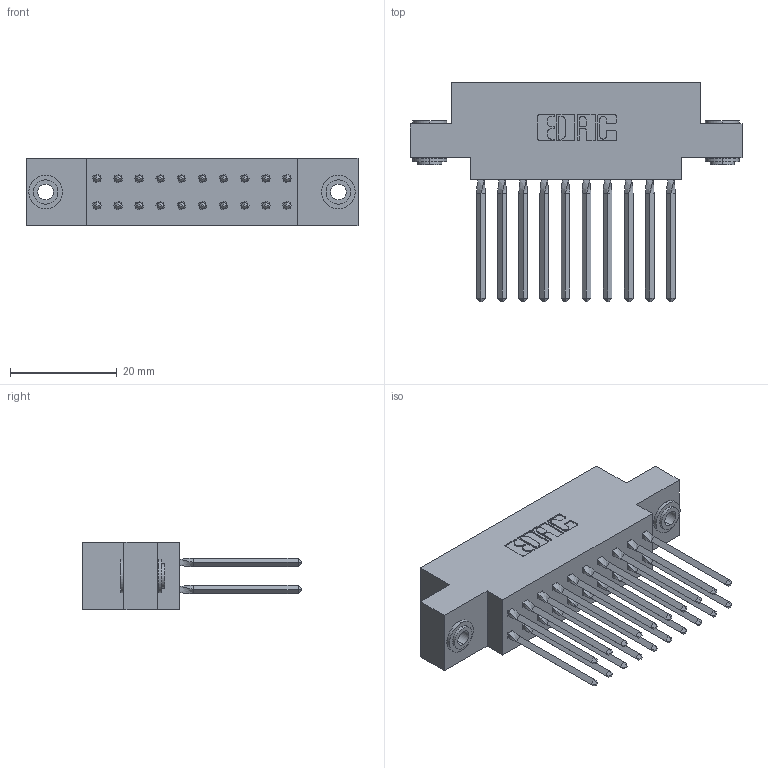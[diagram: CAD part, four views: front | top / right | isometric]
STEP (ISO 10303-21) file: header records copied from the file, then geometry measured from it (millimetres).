
FILE_DESCRIPTION (( 'STEP AP203' ), '1' );
FILE_NAME ('317-020-543-803.STEP', '2020-02-27T16:52:11', ( '' ), ( '' ), 'SwSTEP 2.0', 'SolidWorks 2016', '' );
FILE_SCHEMA (( 'CONFIG_CONTROL_DESIGN' ));
Length unit declared in the file: inch
Products named in the file (4): 317 Part_.156 Dia - TH; 317-290-001_543; 345-250-002_345-250-002-102; 317-020-543-803
Assembly tree (23 placements, depth 2):
  317-020-543-803
    317 Part_.156 Dia - TH
    317-290-001_543  x20
    345-250-002_345-250-002-102  x2
Bounding box: 62.33 x 41.15 x 12.7 mm (x, y, z)
Volume: 9498.2 mm3; surface area: 13365.4 mm2
Topology: 23 solids, 23 shells, 1920 faces, 5291 edges, 3410 vertices
Faces by surface type: plane 1528, cylinder 304, bspline 80, cone 8
Entity records: 19569 total; most frequent: CARTESIAN_POINT 3794, ORIENTED_EDGE 3286, DIRECTION 2787, EDGE_CURVE 1643, VECTOR 1363, LINE 1363, VERTEX_POINT 1087, AXIS2_PLACEMENT_3D 712
